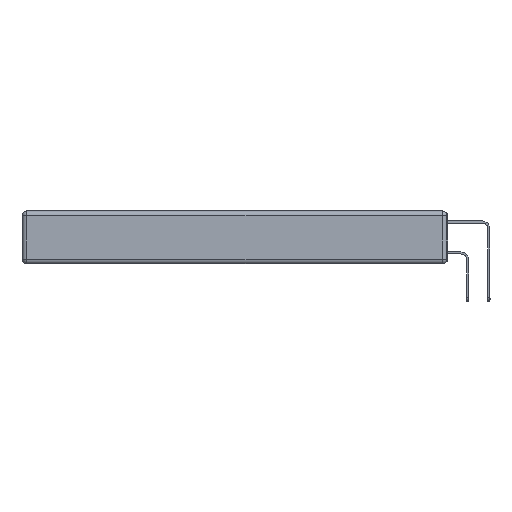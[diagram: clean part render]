
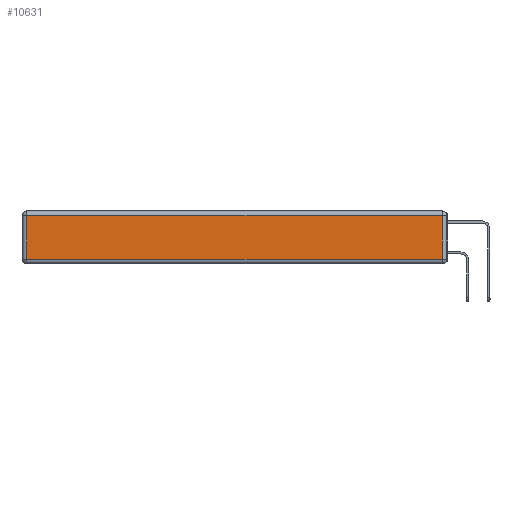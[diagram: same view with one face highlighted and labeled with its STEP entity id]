
A CAD part, left-side view. The second image highlights one B-rep face of the part: STEP entity #10631.
In plain terms, the highlighted planar face has unit normal (-1, 0, 0).
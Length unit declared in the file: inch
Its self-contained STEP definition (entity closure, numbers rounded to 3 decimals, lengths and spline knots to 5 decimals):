
#569 = ORIENTED_EDGE ( 'NONE', *, *, #17396, .T. ) ;
#2034 = VERTEX_POINT ( 'NONE', #15360 ) ;
#2793 = PLANE ( 'NONE',  #6489 ) ;
#3018 = VECTOR ( 'NONE', #8657, 39.37008 ) ;
#4037 = LINE ( 'NONE', #7052, #18654 ) ;
#4214 = ORIENTED_EDGE ( 'NONE', *, *, #6460, .T. ) ;
#4715 = CARTESIAN_POINT ( 'NONE',  ( 0., 2.72, -0.313 ) ) ;
#5226 = VERTEX_POINT ( 'NONE', #18652 ) ;
#5355 = EDGE_CURVE ( 'NONE', #10171, #10602, #9923, .T. ) ;
#5607 = VECTOR ( 'NONE', #14227, 39.37008 ) ;
#6460 = EDGE_CURVE ( 'NONE', #2034, #5226, #4037, .T. ) ;
#6489 = AXIS2_PLACEMENT_3D ( 'NONE', #18375, #13856, #9001 ) ;
#6683 = ORIENTED_EDGE ( 'NONE', *, *, #5355, .T. ) ;
#6923 = FACE_OUTER_BOUND ( 'NONE', #14095, .T. ) ;
#7052 = CARTESIAN_POINT ( 'NONE',  ( 0., 0.03, -0.343 ) ) ;
#7691 = LINE ( 'NONE', #18079, #20015 ) ;
#8657 = DIRECTION ( 'NONE',  ( 0., -1., 0. ) ) ;
#9001 = DIRECTION ( 'NONE',  ( 0., 0., 1. ) ) ;
#9923 = LINE ( 'NONE', #14362, #5607 ) ;
#10171 = VERTEX_POINT ( 'NONE', #16856 ) ;
#10602 = VERTEX_POINT ( 'NONE', #4715 ) ;
#10631 = ADVANCED_FACE ( 'NONE', ( #6923 ), #2793, .T. ) ;
#11838 = CARTESIAN_POINT ( 'NONE',  ( 0., 0., -0.313 ) ) ;
#13684 = EDGE_CURVE ( 'NONE', #10602, #2034, #17411, .T. ) ;
#13856 = DIRECTION ( 'NONE',  ( -1., 0., 0. ) ) ;
#14095 = EDGE_LOOP ( 'NONE', ( #20825, #4214, #569, #6683 ) ) ;
#14227 = DIRECTION ( 'NONE',  ( 0., 0., -1. ) ) ;
#14362 = CARTESIAN_POINT ( 'NONE',  ( 0., 2.72, -0.343 ) ) ;
#15360 = CARTESIAN_POINT ( 'NONE',  ( 0., 0.03, -0.313 ) ) ;
#16631 = DIRECTION ( 'NONE',  ( 0., 0., 1. ) ) ;
#16856 = CARTESIAN_POINT ( 'NONE',  ( 0., 2.72, -0.03 ) ) ;
#17396 = EDGE_CURVE ( 'NONE', #5226, #10171, #7691, .T. ) ;
#17411 = LINE ( 'NONE', #11838, #3018 ) ;
#18079 = CARTESIAN_POINT ( 'NONE',  ( 0., 2.75, -0.03 ) ) ;
#18151 = DIRECTION ( 'NONE',  ( 0., 1., 0. ) ) ;
#18375 = CARTESIAN_POINT ( 'NONE',  ( 0., 0., -0.343 ) ) ;
#18652 = CARTESIAN_POINT ( 'NONE',  ( 0., 0.03, -0.03 ) ) ;
#18654 = VECTOR ( 'NONE', #16631, 39.37008 ) ;
#20015 = VECTOR ( 'NONE', #18151, 39.37008 ) ;
#20825 = ORIENTED_EDGE ( 'NONE', *, *, #13684, .T. ) ;
